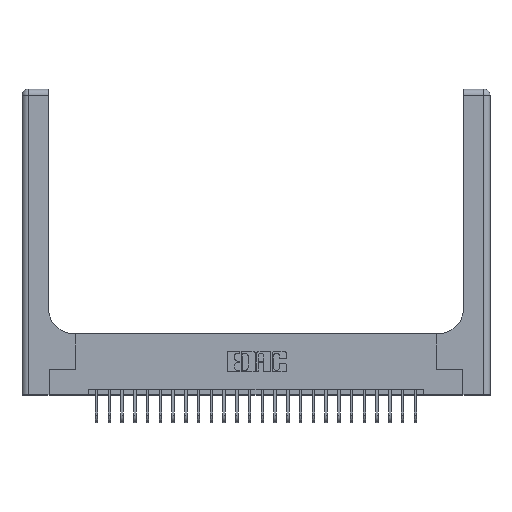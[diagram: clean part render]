
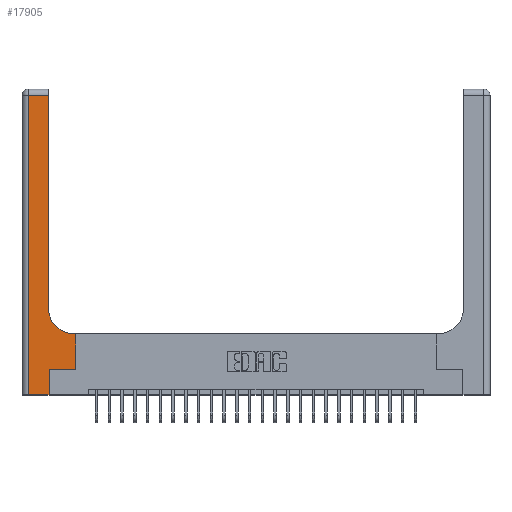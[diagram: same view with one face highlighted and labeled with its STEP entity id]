
A CAD part, top view. The second image highlights one B-rep face of the part: STEP entity #17905.
In plain terms, the highlighted planar face has unit normal (0, 0, 1).
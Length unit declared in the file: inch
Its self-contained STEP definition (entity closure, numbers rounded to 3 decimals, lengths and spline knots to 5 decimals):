
#96 = CIRCLE ( 'NONE', #7640, 0.25 ) ;
#149 = CARTESIAN_POINT ( 'NONE',  ( 0.265, 0.25, 0.37 ) ) ;
#663 = LINE ( 'NONE', #8970, #12487 ) ;
#680 = VECTOR ( 'NONE', #4986, 39.37008 ) ;
#915 = DIRECTION ( 'NONE',  ( -1., 0., 0. ) ) ;
#1082 = ORIENTED_EDGE ( 'NONE', *, *, #1934, .T. ) ;
#1108 = CARTESIAN_POINT ( 'NONE',  ( 0.528, 0.25, 0.37 ) ) ;
#1268 = DIRECTION ( 'NONE',  ( 0., 0., -1. ) ) ;
#1784 = LINE ( 'NONE', #16615, #6881 ) ;
#1796 = CARTESIAN_POINT ( 'NONE',  ( 0.06, 3., 0.37 ) ) ;
#1934 = EDGE_CURVE ( 'NONE', #6050, #24295, #16246, .T. ) ;
#1968 = EDGE_CURVE ( 'NONE', #15648, #6050, #5164, .T. ) ;
#2123 = ORIENTED_EDGE ( 'NONE', *, *, #1968, .T. ) ;
#2517 = CARTESIAN_POINT ( 'NONE',  ( 0.265, 0., 0.37 ) ) ;
#2997 = EDGE_CURVE ( 'NONE', #10748, #8426, #7099, .T. ) ;
#3028 = CARTESIAN_POINT ( 'NONE',  ( 0.26, 0.85, 0.37 ) ) ;
#3095 = VERTEX_POINT ( 'NONE', #17470 ) ;
#3149 = CARTESIAN_POINT ( 'NONE',  ( 0.265, 0.25, 0.37 ) ) ;
#3592 = DIRECTION ( 'NONE',  ( 0., -1., 0. ) ) ;
#3866 = ORIENTED_EDGE ( 'NONE', *, *, #15919, .T. ) ;
#4684 = ORIENTED_EDGE ( 'NONE', *, *, #25764, .T. ) ;
#4986 = DIRECTION ( 'NONE',  ( 0., 1., 0. ) ) ;
#5013 = CARTESIAN_POINT ( 'NONE',  ( 0.51, 0.85, 0.37 ) ) ;
#5110 = VERTEX_POINT ( 'NONE', #9296 ) ;
#5164 = LINE ( 'NONE', #17532, #680 ) ;
#5246 = VERTEX_POINT ( 'NONE', #25572 ) ;
#5466 = VECTOR ( 'NONE', #19655, 39.37008 ) ;
#6050 = VERTEX_POINT ( 'NONE', #23915 ) ;
#6467 = VECTOR ( 'NONE', #15137, 39.37008 ) ;
#6819 = CARTESIAN_POINT ( 'NONE',  ( 0., 3., 0.37 ) ) ;
#6881 = VECTOR ( 'NONE', #22749, 39.37008 ) ;
#7099 = LINE ( 'NONE', #22822, #6467 ) ;
#7640 = AXIS2_PLACEMENT_3D ( 'NONE', #5013, #1268, #23250 ) ;
#8305 = DIRECTION ( 'NONE',  ( 1., 0., 0. ) ) ;
#8426 = VERTEX_POINT ( 'NONE', #12662 ) ;
#8970 = CARTESIAN_POINT ( 'NONE',  ( 0.26, 0.6, 0.37 ) ) ;
#8994 = LINE ( 'NONE', #2517, #15663 ) ;
#9296 = CARTESIAN_POINT ( 'NONE',  ( 0.51, 0.6, 0.37 ) ) ;
#9887 = ORIENTED_EDGE ( 'NONE', *, *, #17034, .T. ) ;
#10305 = ORIENTED_EDGE ( 'NONE', *, *, #20207, .T. ) ;
#10354 = CARTESIAN_POINT ( 'NONE',  ( 0.06, 2.94, 0.37 ) ) ;
#10729 = DIRECTION ( 'NONE',  ( 0., 1., 0. ) ) ;
#10748 = VERTEX_POINT ( 'NONE', #1108 ) ;
#10881 = CARTESIAN_POINT ( 'NONE',  ( 0., 2.94, 0.37 ) ) ;
#11343 = VECTOR ( 'NONE', #3592, 39.37008 ) ;
#11481 = ORIENTED_EDGE ( 'NONE', *, *, #20130, .T. ) ;
#11647 = LINE ( 'NONE', #1796, #11343 ) ;
#12487 = VECTOR ( 'NONE', #25079, 39.37008 ) ;
#12662 = CARTESIAN_POINT ( 'NONE',  ( 0.528, 0.6, 0.37 ) ) ;
#13685 = EDGE_LOOP ( 'NONE', ( #2123, #1082, #10305, #11481, #3866, #4684, #24614, #9887, #20269 ) ) ;
#14130 = LINE ( 'NONE', #149, #25013 ) ;
#14763 = EDGE_CURVE ( 'NONE', #5110, #15648, #96, .T. ) ;
#15137 = DIRECTION ( 'NONE',  ( 0., 1., 0. ) ) ;
#15648 = VERTEX_POINT ( 'NONE', #3028 ) ;
#15663 = VECTOR ( 'NONE', #10729, 39.37008 ) ;
#15919 = EDGE_CURVE ( 'NONE', #5246, #19534, #8994, .T. ) ;
#16246 = LINE ( 'NONE', #10881, #5466 ) ;
#16615 = CARTESIAN_POINT ( 'NONE',  ( 0., 0., 0.37 ) ) ;
#17034 = EDGE_CURVE ( 'NONE', #8426, #5110, #663, .T. ) ;
#17116 = FACE_OUTER_BOUND ( 'NONE', #13685, .T. ) ;
#17470 = CARTESIAN_POINT ( 'NONE',  ( 0.06, 0., 0.37 ) ) ;
#17532 = CARTESIAN_POINT ( 'NONE',  ( 0.26, 3., 0.37 ) ) ;
#17905 = ADVANCED_FACE ( 'NONE', ( #17116 ), #18929, .F. ) ;
#18929 = PLANE ( 'NONE',  #21161 ) ;
#19534 = VERTEX_POINT ( 'NONE', #3149 ) ;
#19655 = DIRECTION ( 'NONE',  ( -1., 0., 0. ) ) ;
#20130 = EDGE_CURVE ( 'NONE', #3095, #5246, #1784, .T. ) ;
#20207 = EDGE_CURVE ( 'NONE', #24295, #3095, #11647, .T. ) ;
#20269 = ORIENTED_EDGE ( 'NONE', *, *, #14763, .T. ) ;
#21161 = AXIS2_PLACEMENT_3D ( 'NONE', #6819, #24901, #915 ) ;
#22749 = DIRECTION ( 'NONE',  ( 1., 0., 0. ) ) ;
#22822 = CARTESIAN_POINT ( 'NONE',  ( 0.528, 0.25, 0.37 ) ) ;
#23250 = DIRECTION ( 'NONE',  ( 1., 0., 0. ) ) ;
#23915 = CARTESIAN_POINT ( 'NONE',  ( 0.26, 2.94, 0.37 ) ) ;
#24295 = VERTEX_POINT ( 'NONE', #10354 ) ;
#24614 = ORIENTED_EDGE ( 'NONE', *, *, #2997, .T. ) ;
#24901 = DIRECTION ( 'NONE',  ( 0., 0., -1. ) ) ;
#25013 = VECTOR ( 'NONE', #8305, 39.37008 ) ;
#25079 = DIRECTION ( 'NONE',  ( -1., 0., 0. ) ) ;
#25572 = CARTESIAN_POINT ( 'NONE',  ( 0.265, 0., 0.37 ) ) ;
#25764 = EDGE_CURVE ( 'NONE', #19534, #10748, #14130, .T. ) ;
